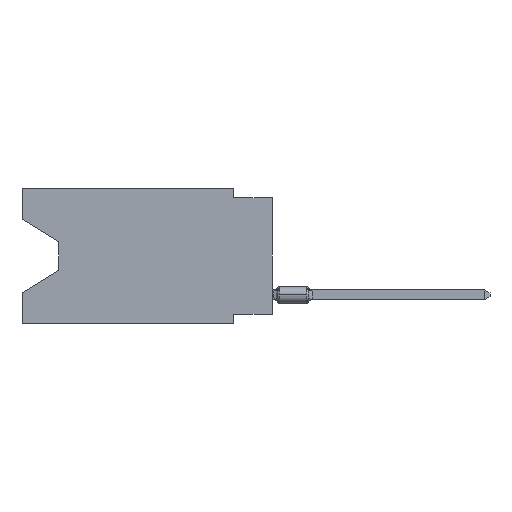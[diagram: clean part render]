
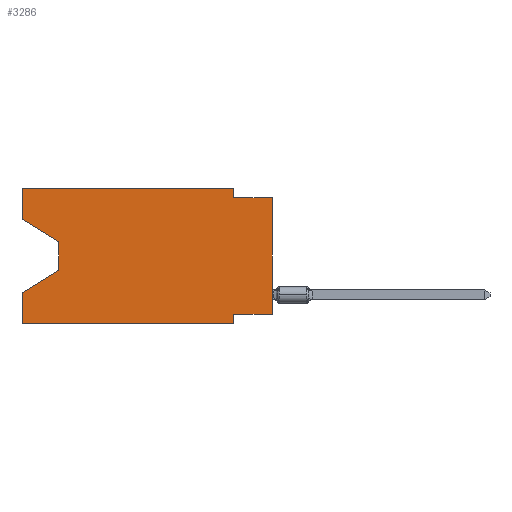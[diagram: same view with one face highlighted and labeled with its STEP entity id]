
A CAD part, left-side view. The second image highlights one B-rep face of the part: STEP entity #3286.
In plain terms, the highlighted planar face has unit normal (-1, 0, 0).
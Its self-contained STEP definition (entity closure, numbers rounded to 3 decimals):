
#36 = DIRECTION ( 'NONE',  ( 0., 0., -1. ) ) ;
#138 = ORIENTED_EDGE ( 'NONE', *, *, #2531, .F. ) ;
#251 = CARTESIAN_POINT ( 'NONE',  ( 0., 0., 0. ) ) ;
#264 = CARTESIAN_POINT ( 'NONE',  ( 0., 16.383, 0. ) ) ;
#535 = DIRECTION ( 'NONE',  ( 0., 0., -1. ) ) ;
#663 = VERTEX_POINT ( 'NONE', #6839 ) ;
#673 = EDGE_CURVE ( 'NONE', #10724, #12718, #5548, .T. ) ;
#758 = CARTESIAN_POINT ( 'NONE',  ( 0., 13.97, -5.385 ) ) ;
#973 = ORIENTED_EDGE ( 'NONE', *, *, #5615, .T. ) ;
#1342 = DIRECTION ( 'NONE',  ( 0., 0., 1. ) ) ;
#1782 = EDGE_CURVE ( 'NONE', #17448, #15101, #4637, .T. ) ;
#1922 = LINE ( 'NONE', #8482, #13835 ) ;
#2426 = EDGE_CURVE ( 'NONE', #12718, #5173, #1922, .T. ) ;
#2531 = EDGE_CURVE ( 'NONE', #15101, #663, #20693, .T. ) ;
#2687 = CARTESIAN_POINT ( 'NONE',  ( 0., 16.383, 0. ) ) ;
#2938 = EDGE_CURVE ( 'NONE', #663, #7439, #10758, .T. ) ;
#3286 = ADVANCED_FACE ( 'NONE', ( #12666 ), #5910, .F. ) ;
#3462 = DIRECTION ( 'NONE',  ( 0., 0., 1. ) ) ;
#3606 = CARTESIAN_POINT ( 'NONE',  ( 0., 0., -8.255 ) ) ;
#3960 = LINE ( 'NONE', #7296, #10546 ) ;
#4214 = ORIENTED_EDGE ( 'NONE', *, *, #11112, .T. ) ;
#4637 = LINE ( 'NONE', #12787, #19607 ) ;
#4659 = AXIS2_PLACEMENT_3D ( 'NONE', #2687, #19096, #15771 ) ;
#4874 = CARTESIAN_POINT ( 'NONE',  ( 0., 2.54, 0. ) ) ;
#5173 = VERTEX_POINT ( 'NONE', #14993 ) ;
#5223 = CARTESIAN_POINT ( 'NONE',  ( 0., 13.97, -3.505 ) ) ;
#5468 = VECTOR ( 'NONE', #10257, 1000. ) ;
#5548 = LINE ( 'NONE', #3606, #21050 ) ;
#5615 = EDGE_CURVE ( 'NONE', #12149, #14863, #13583, .T. ) ;
#5910 = PLANE ( 'NONE',  #4659 ) ;
#6485 = CARTESIAN_POINT ( 'NONE',  ( 0., 13.97, -3.505 ) ) ;
#6568 = DIRECTION ( 'NONE',  ( 0., -1., 0. ) ) ;
#6708 = CARTESIAN_POINT ( 'NONE',  ( 0., 16.383, -6.852 ) ) ;
#6778 = LINE ( 'NONE', #10097, #11910 ) ;
#6784 = ORIENTED_EDGE ( 'NONE', *, *, #673, .F. ) ;
#6839 = CARTESIAN_POINT ( 'NONE',  ( 0., 2.54, -0.635 ) ) ;
#7296 = CARTESIAN_POINT ( 'NONE',  ( 0., 16.383, 0. ) ) ;
#7439 = VERTEX_POINT ( 'NONE', #10201 ) ;
#8083 = VECTOR ( 'NONE', #11188, 1000. ) ;
#8393 = DIRECTION ( 'NONE',  ( 0., -1., 0. ) ) ;
#8461 = ORIENTED_EDGE ( 'NONE', *, *, #2426, .F. ) ;
#8482 = CARTESIAN_POINT ( 'NONE',  ( 0., 2.54, -8.89 ) ) ;
#8495 = EDGE_LOOP ( 'NONE', ( #973, #20665, #10434, #19888, #9079, #8461, #6784, #4214, #16283, #138, #13453, #15252 ) ) ;
#8563 = DIRECTION ( 'NONE',  ( 0., 1., 0. ) ) ;
#8603 = DIRECTION ( 'NONE',  ( 0., 0.855, -0.519 ) ) ;
#8624 = LINE ( 'NONE', #251, #10603 ) ;
#8697 = EDGE_CURVE ( 'NONE', #12684, #18668, #3960, .T. ) ;
#9079 = ORIENTED_EDGE ( 'NONE', *, *, #16252, .T. ) ;
#9259 = CARTESIAN_POINT ( 'NONE',  ( 0., 0., -0.635 ) ) ;
#9898 = VERTEX_POINT ( 'NONE', #11835 ) ;
#10097 = CARTESIAN_POINT ( 'NONE',  ( 0., 16.383, -8.89 ) ) ;
#10201 = CARTESIAN_POINT ( 'NONE',  ( 0., 0., -0.635 ) ) ;
#10257 = DIRECTION ( 'NONE',  ( 0., -0.855, -0.519 ) ) ;
#10434 = ORIENTED_EDGE ( 'NONE', *, *, #14015, .T. ) ;
#10546 = VECTOR ( 'NONE', #18563, 1000. ) ;
#10603 = VECTOR ( 'NONE', #3462, 1000. ) ;
#10724 = VERTEX_POINT ( 'NONE', #20013 ) ;
#10726 = VECTOR ( 'NONE', #18852, 1000. ) ;
#10758 = LINE ( 'NONE', #9259, #8083 ) ;
#11112 = EDGE_CURVE ( 'NONE', #10724, #7439, #8624, .T. ) ;
#11188 = DIRECTION ( 'NONE',  ( 0., -1., 0. ) ) ;
#11835 = CARTESIAN_POINT ( 'NONE',  ( 0., 13.97, -5.385 ) ) ;
#11870 = CARTESIAN_POINT ( 'NONE',  ( 0., 16.383, -2.038 ) ) ;
#11910 = VECTOR ( 'NONE', #8393, 1000. ) ;
#12136 = EDGE_CURVE ( 'NONE', #14863, #9898, #21069, .T. ) ;
#12149 = VERTEX_POINT ( 'NONE', #21176 ) ;
#12300 = VECTOR ( 'NONE', #36, 1000. ) ;
#12644 = CARTESIAN_POINT ( 'NONE',  ( 0., 2.54, 0. ) ) ;
#12666 = FACE_OUTER_BOUND ( 'NONE', #8495, .T. ) ;
#12684 = VERTEX_POINT ( 'NONE', #19528 ) ;
#12718 = VERTEX_POINT ( 'NONE', #13098 ) ;
#12787 = CARTESIAN_POINT ( 'NONE',  ( 0., 16.383, 0. ) ) ;
#13098 = CARTESIAN_POINT ( 'NONE',  ( 0., 2.54, -8.255 ) ) ;
#13453 = ORIENTED_EDGE ( 'NONE', *, *, #1782, .F. ) ;
#13583 = LINE ( 'NONE', #11870, #5468 ) ;
#13835 = VECTOR ( 'NONE', #535, 1000. ) ;
#14015 = EDGE_CURVE ( 'NONE', #9898, #18668, #16747, .T. ) ;
#14111 = CARTESIAN_POINT ( 'NONE',  ( 0., 16.383, 0. ) ) ;
#14863 = VERTEX_POINT ( 'NONE', #5223 ) ;
#14993 = CARTESIAN_POINT ( 'NONE',  ( 0., 2.54, -8.89 ) ) ;
#15101 = VERTEX_POINT ( 'NONE', #4874 ) ;
#15252 = ORIENTED_EDGE ( 'NONE', *, *, #17397, .F. ) ;
#15679 = VECTOR ( 'NONE', #1342, 1000. ) ;
#15771 = DIRECTION ( 'NONE',  ( 0., 0., -1. ) ) ;
#15941 = VECTOR ( 'NONE', #8603, 1000. ) ;
#16252 = EDGE_CURVE ( 'NONE', #12684, #5173, #6778, .T. ) ;
#16283 = ORIENTED_EDGE ( 'NONE', *, *, #2938, .F. ) ;
#16747 = LINE ( 'NONE', #758, #15941 ) ;
#17397 = EDGE_CURVE ( 'NONE', #12149, #17448, #17651, .T. ) ;
#17448 = VERTEX_POINT ( 'NONE', #264 ) ;
#17651 = LINE ( 'NONE', #14111, #15679 ) ;
#18563 = DIRECTION ( 'NONE',  ( 0., 0., 1. ) ) ;
#18668 = VERTEX_POINT ( 'NONE', #6708 ) ;
#18852 = DIRECTION ( 'NONE',  ( 0., 0., -1. ) ) ;
#19096 = DIRECTION ( 'NONE',  ( 1., 0., 0. ) ) ;
#19528 = CARTESIAN_POINT ( 'NONE',  ( 0., 16.383, -8.89 ) ) ;
#19607 = VECTOR ( 'NONE', #6568, 1000. ) ;
#19888 = ORIENTED_EDGE ( 'NONE', *, *, #8697, .F. ) ;
#20013 = CARTESIAN_POINT ( 'NONE',  ( 0., 0., -8.255 ) ) ;
#20665 = ORIENTED_EDGE ( 'NONE', *, *, #12136, .T. ) ;
#20693 = LINE ( 'NONE', #12644, #10726 ) ;
#21050 = VECTOR ( 'NONE', #8563, 1000. ) ;
#21069 = LINE ( 'NONE', #6485, #12300 ) ;
#21176 = CARTESIAN_POINT ( 'NONE',  ( 0., 16.383, -2.038 ) ) ;
